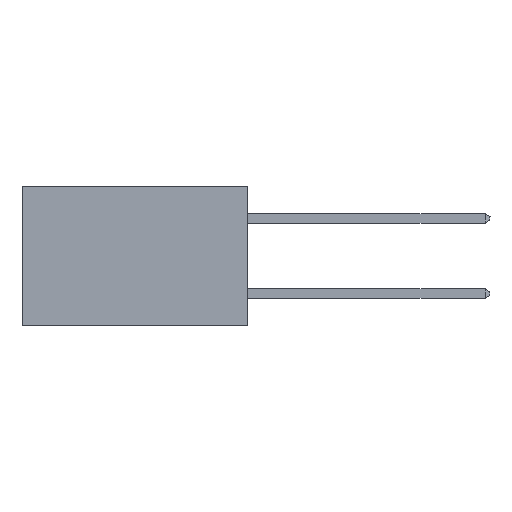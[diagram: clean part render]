
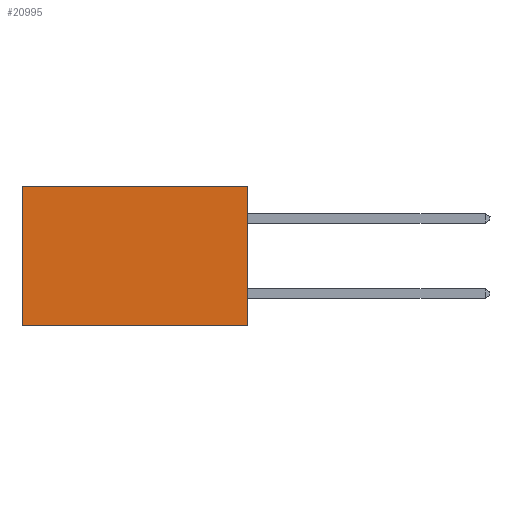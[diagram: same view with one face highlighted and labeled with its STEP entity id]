
A CAD part, left-side view. The second image highlights one B-rep face of the part: STEP entity #20995.
In plain terms, the highlighted planar face has unit normal (-1, 0, 0).
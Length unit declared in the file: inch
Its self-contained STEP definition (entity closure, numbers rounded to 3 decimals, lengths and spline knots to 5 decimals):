
#111 = CARTESIAN_POINT ( 'NONE',  ( 0.2615, 0.6, 0. ) ) ;
#456 = ORIENTED_EDGE ( 'NONE', *, *, #16139, .T. ) ;
#1279 = VECTOR ( 'NONE', #20428, 39.37008 ) ;
#1659 = ORIENTED_EDGE ( 'NONE', *, *, #2506, .F. ) ;
#2028 = AXIS2_PLACEMENT_3D ( 'NONE', #14159, #12410, #6041 ) ;
#2506 = EDGE_CURVE ( 'NONE', #13358, #15694, #5608, .T. ) ;
#3284 = DIRECTION ( 'NONE',  ( 0., 0., -1. ) ) ;
#3338 = LINE ( 'NONE', #14854, #12265 ) ;
#3765 = EDGE_LOOP ( 'NONE', ( #456, #1659, #17360, #8030 ) ) ;
#4291 = FACE_OUTER_BOUND ( 'NONE', #3765, .T. ) ;
#4930 = CARTESIAN_POINT ( 'NONE',  ( 0.2615, 0.6, -0.37 ) ) ;
#5608 = LINE ( 'NONE', #13821, #1279 ) ;
#6041 = DIRECTION ( 'NONE',  ( 0., 0., -1. ) ) ;
#6961 = DIRECTION ( 'NONE',  ( 0., 0., -1. ) ) ;
#7143 = CARTESIAN_POINT ( 'NONE',  ( 0.2615, 0.6, -0.37 ) ) ;
#7693 = PLANE ( 'NONE',  #2028 ) ;
#7932 = CARTESIAN_POINT ( 'NONE',  ( 0.2615, 0., 0. ) ) ;
#8030 = ORIENTED_EDGE ( 'NONE', *, *, #14055, .T. ) ;
#8667 = LINE ( 'NONE', #4930, #14865 ) ;
#9810 = VECTOR ( 'NONE', #17563, 39.37008 ) ;
#10885 = LINE ( 'NONE', #21190, #9810 ) ;
#12265 = VECTOR ( 'NONE', #6961, 39.37008 ) ;
#12410 = DIRECTION ( 'NONE',  ( 1., 0., 0. ) ) ;
#13358 = VERTEX_POINT ( 'NONE', #18819 ) ;
#13821 = CARTESIAN_POINT ( 'NONE',  ( 0.2615, 0., -0.37 ) ) ;
#14055 = EDGE_CURVE ( 'NONE', #17494, #16595, #10885, .T. ) ;
#14159 = CARTESIAN_POINT ( 'NONE',  ( 0.2615, 0., -0.37 ) ) ;
#14680 = EDGE_CURVE ( 'NONE', #17494, #13358, #3338, .T. ) ;
#14854 = CARTESIAN_POINT ( 'NONE',  ( 0.2615, 0., -0.37 ) ) ;
#14865 = VECTOR ( 'NONE', #3284, 39.37008 ) ;
#15694 = VERTEX_POINT ( 'NONE', #7143 ) ;
#16139 = EDGE_CURVE ( 'NONE', #16595, #15694, #8667, .T. ) ;
#16595 = VERTEX_POINT ( 'NONE', #111 ) ;
#17360 = ORIENTED_EDGE ( 'NONE', *, *, #14680, .F. ) ;
#17494 = VERTEX_POINT ( 'NONE', #7932 ) ;
#17563 = DIRECTION ( 'NONE',  ( 0., 1., 0. ) ) ;
#18819 = CARTESIAN_POINT ( 'NONE',  ( 0.2615, 0., -0.37 ) ) ;
#20428 = DIRECTION ( 'NONE',  ( 0., 1., 0. ) ) ;
#20995 = ADVANCED_FACE ( 'NONE', ( #4291 ), #7693, .F. ) ;
#21190 = CARTESIAN_POINT ( 'NONE',  ( 0.2615, 0., 0. ) ) ;
